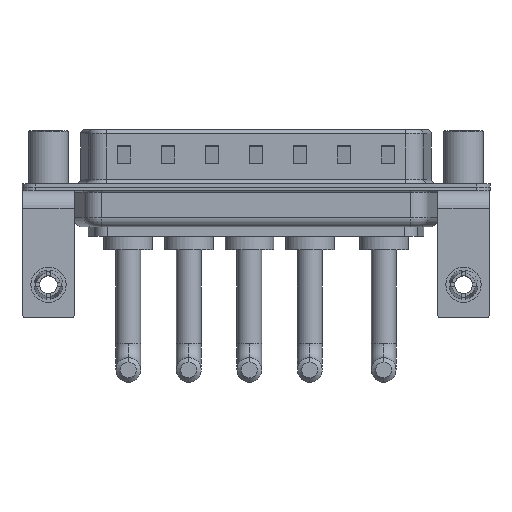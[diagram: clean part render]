
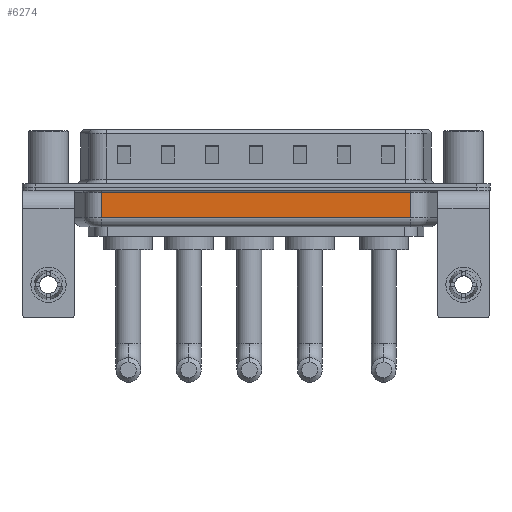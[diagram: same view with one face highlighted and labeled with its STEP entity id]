
A CAD part, front view. The second image highlights one B-rep face of the part: STEP entity #6274.
In plain terms, the highlighted planar face has unit normal (0, -1, 0).
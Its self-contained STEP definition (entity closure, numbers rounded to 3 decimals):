
#83 = VERTEX_POINT ( 'NONE', #14160 ) ;
#109 = VECTOR ( 'NONE', #7270, 1000. ) ;
#449 = VERTEX_POINT ( 'NONE', #17866 ) ;
#818 = ORIENTED_EDGE ( 'NONE', *, *, #1359, .T. ) ;
#1359 = EDGE_CURVE ( 'NONE', #449, #12737, #3909, .T. ) ;
#2510 = EDGE_CURVE ( 'NONE', #83, #9218, #5359, .T. ) ;
#2837 = LINE ( 'NONE', #15523, #109 ) ;
#3592 = VECTOR ( 'NONE', #6444, 1000. ) ;
#3791 = DIRECTION ( 'NONE',  ( 0., 1., 0. ) ) ;
#3909 = LINE ( 'NONE', #5717, #13249 ) ;
#4748 = ORIENTED_EDGE ( 'NONE', *, *, #2510, .T. ) ;
#4996 = CARTESIAN_POINT ( 'NONE',  ( 6.006, -5.35, -4.5 ) ) ;
#5359 = LINE ( 'NONE', #13879, #12129 ) ;
#5717 = CARTESIAN_POINT ( 'NONE',  ( 6.006, -5.35, -0.65 ) ) ;
#5811 = ORIENTED_EDGE ( 'NONE', *, *, #16865, .T. ) ;
#6274 = ADVANCED_FACE ( 'NONE', ( #9148 ), #13054, .F. ) ;
#6444 = DIRECTION ( 'NONE',  ( 0., 0., 1. ) ) ;
#6978 = DIRECTION ( 'NONE',  ( -1., 0., 0. ) ) ;
#7270 = DIRECTION ( 'NONE',  ( 0., 0., 1. ) ) ;
#9148 = FACE_OUTER_BOUND ( 'NONE', #15880, .T. ) ;
#9218 = VERTEX_POINT ( 'NONE', #17438 ) ;
#10599 = CARTESIAN_POINT ( 'NONE',  ( 6.006, -5.35, -4.5 ) ) ;
#10895 = DIRECTION ( 'NONE',  ( 1., 0., 0. ) ) ;
#12129 = VECTOR ( 'NONE', #10895, 1000. ) ;
#12697 = CARTESIAN_POINT ( 'NONE',  ( 6.006, -5.35, -0.65 ) ) ;
#12737 = VERTEX_POINT ( 'NONE', #12697 ) ;
#13054 = PLANE ( 'NONE',  #13737 ) ;
#13249 = VECTOR ( 'NONE', #6978, 1000. ) ;
#13737 = AXIS2_PLACEMENT_3D ( 'NONE', #10599, #3791, #15868 ) ;
#13879 = CARTESIAN_POINT ( 'NONE',  ( 6.006, -5.35, -3.5 ) ) ;
#14160 = CARTESIAN_POINT ( 'NONE',  ( 6.006, -5.35, -3.5 ) ) ;
#15523 = CARTESIAN_POINT ( 'NONE',  ( 41.044, -5.35, -4.5 ) ) ;
#15868 = DIRECTION ( 'NONE',  ( 0., 0., 1. ) ) ;
#15880 = EDGE_LOOP ( 'NONE', ( #17249, #4748, #5811, #818 ) ) ;
#16416 = LINE ( 'NONE', #4996, #3592 ) ;
#16865 = EDGE_CURVE ( 'NONE', #9218, #449, #2837, .T. ) ;
#17195 = EDGE_CURVE ( 'NONE', #83, #12737, #16416, .T. ) ;
#17249 = ORIENTED_EDGE ( 'NONE', *, *, #17195, .F. ) ;
#17438 = CARTESIAN_POINT ( 'NONE',  ( 41.044, -5.35, -3.5 ) ) ;
#17866 = CARTESIAN_POINT ( 'NONE',  ( 41.044, -5.35, -0.65 ) ) ;
